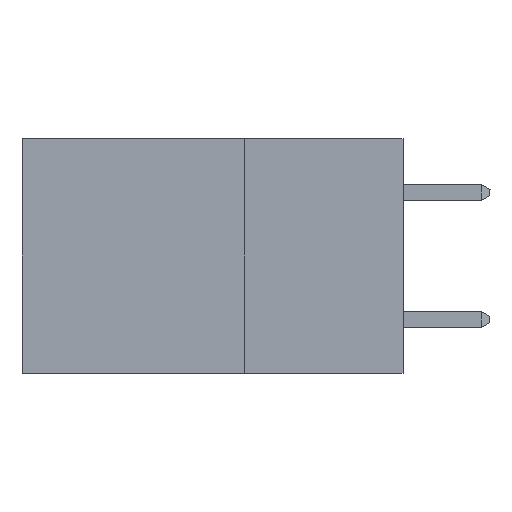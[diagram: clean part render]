
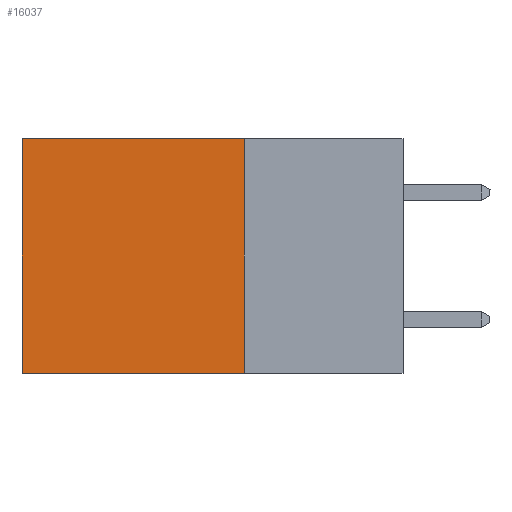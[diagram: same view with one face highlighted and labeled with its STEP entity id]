
A CAD part, left-side view. The second image highlights one B-rep face of the part: STEP entity #16037.
In plain terms, the highlighted planar face has unit normal (-1, 0, 0).
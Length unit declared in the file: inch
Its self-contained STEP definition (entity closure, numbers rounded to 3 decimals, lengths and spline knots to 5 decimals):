
#238 = CARTESIAN_POINT ( 'NONE',  ( 0.2875, 0.25, 0. ) ) ;
#677 = LINE ( 'NONE', #16634, #2164 ) ;
#1390 = PLANE ( 'NONE',  #4596 ) ;
#1797 = DIRECTION ( 'NONE',  ( 0., 1., 0. ) ) ;
#1836 = VERTEX_POINT ( 'NONE', #9603 ) ;
#1895 = DIRECTION ( 'NONE',  ( 0., 0., -1. ) ) ;
#2155 = VERTEX_POINT ( 'NONE', #15825 ) ;
#2164 = VECTOR ( 'NONE', #13531, 39.37008 ) ;
#2871 = ORIENTED_EDGE ( 'NONE', *, *, #13907, .F. ) ;
#4233 = VECTOR ( 'NONE', #11384, 39.37008 ) ;
#4596 = AXIS2_PLACEMENT_3D ( 'NONE', #18851, #14100, #17262 ) ;
#5172 = EDGE_CURVE ( 'NONE', #2155, #14995, #16746, .T. ) ;
#5335 = VECTOR ( 'NONE', #1797, 39.37008 ) ;
#6517 = VERTEX_POINT ( 'NONE', #17112 ) ;
#6680 = ORIENTED_EDGE ( 'NONE', *, *, #19934, .T. ) ;
#7349 = VECTOR ( 'NONE', #1895, 39.37008 ) ;
#9496 = LINE ( 'NONE', #238, #4233 ) ;
#9603 = CARTESIAN_POINT ( 'NONE',  ( 0.2875, 0.6, 0. ) ) ;
#10060 = FACE_OUTER_BOUND ( 'NONE', #11436, .T. ) ;
#10157 = EDGE_CURVE ( 'NONE', #2155, #1836, #9496, .T. ) ;
#11384 = DIRECTION ( 'NONE',  ( 0., 1., 0. ) ) ;
#11436 = EDGE_LOOP ( 'NONE', ( #6680, #2871, #16318, #16307 ) ) ;
#13531 = DIRECTION ( 'NONE',  ( 0., 0., -1. ) ) ;
#13907 = EDGE_CURVE ( 'NONE', #14995, #6517, #17246, .T. ) ;
#14100 = DIRECTION ( 'NONE',  ( 1., 0., 0. ) ) ;
#14381 = CARTESIAN_POINT ( 'NONE',  ( 0.2875, 0.25, -0.37 ) ) ;
#14995 = VERTEX_POINT ( 'NONE', #16895 ) ;
#15825 = CARTESIAN_POINT ( 'NONE',  ( 0.2875, 0.25, 0. ) ) ;
#16037 = ADVANCED_FACE ( 'NONE', ( #10060 ), #1390, .F. ) ;
#16307 = ORIENTED_EDGE ( 'NONE', *, *, #10157, .T. ) ;
#16318 = ORIENTED_EDGE ( 'NONE', *, *, #5172, .F. ) ;
#16634 = CARTESIAN_POINT ( 'NONE',  ( 0.2875, 0.6, 0. ) ) ;
#16746 = LINE ( 'NONE', #19424, #7349 ) ;
#16895 = CARTESIAN_POINT ( 'NONE',  ( 0.2875, 0.25, -0.37 ) ) ;
#17112 = CARTESIAN_POINT ( 'NONE',  ( 0.2875, 0.6, -0.37 ) ) ;
#17246 = LINE ( 'NONE', #14381, #5335 ) ;
#17262 = DIRECTION ( 'NONE',  ( 0., 0., -1. ) ) ;
#18851 = CARTESIAN_POINT ( 'NONE',  ( 0.2875, 0.25, 0. ) ) ;
#19424 = CARTESIAN_POINT ( 'NONE',  ( 0.2875, 0.25, 0. ) ) ;
#19934 = EDGE_CURVE ( 'NONE', #1836, #6517, #677, .T. ) ;
